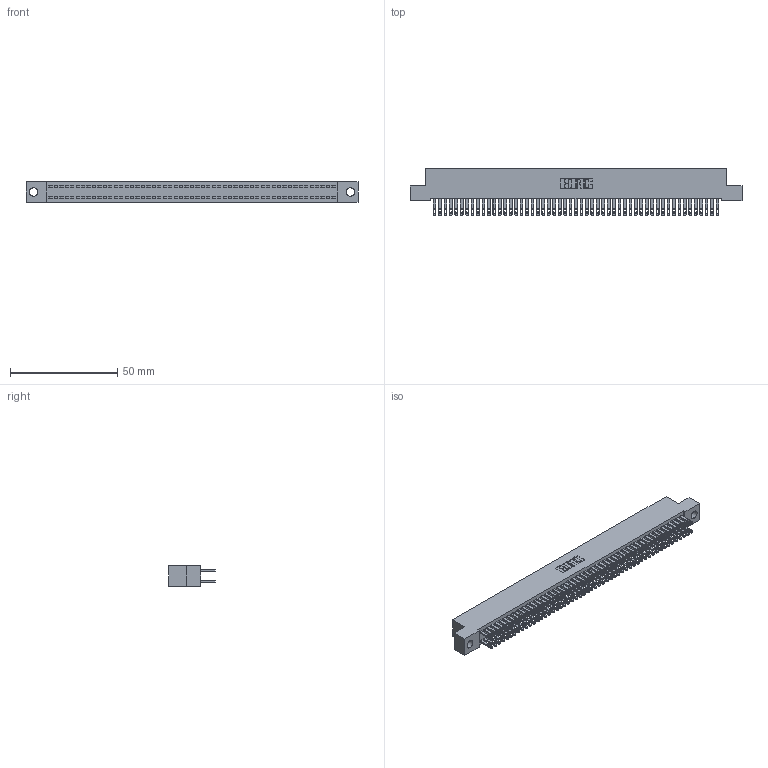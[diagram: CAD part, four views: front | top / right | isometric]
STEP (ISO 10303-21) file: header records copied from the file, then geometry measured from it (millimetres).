
FILE_DESCRIPTION (( 'STEP AP203' ), '1' );
FILE_NAME ('342-106-500-204.STEP', '2019-10-04T19:00:50', ( '' ), ( '' ), 'SwSTEP 2.0', 'SolidWorks 2016', '' );
FILE_SCHEMA (( 'CONFIG_CONTROL_DESIGN' ));
Length unit declared in the file: inch
Products named in the file (3): 345-292-001_345-293-100; 342-106-500-204; 342 Part_.156 TH
Assembly tree (107 placements, depth 2):
  342-106-500-204
    342 Part_.156 TH
    345-292-001_345-293-100  x106
Bounding box: 154.94 x 21.85 x 9.4 mm (x, y, z)
Volume: 14210.3 mm3; surface area: 24240.9 mm2
Topology: 107 solids, 107 shells, 5198 faces, 15881 edges, 10586 vertices
Faces by surface type: plane 3246, cylinder 1952
Entity records: 32475 total; most frequent: CARTESIAN_POINT 5366, ORIENTED_EDGE 5302, DIRECTION 4567, EDGE_CURVE 2651, LINE 2519, VECTOR 2519, VERTEX_POINT 1766, AXIS2_PLACEMENT_3D 1024
